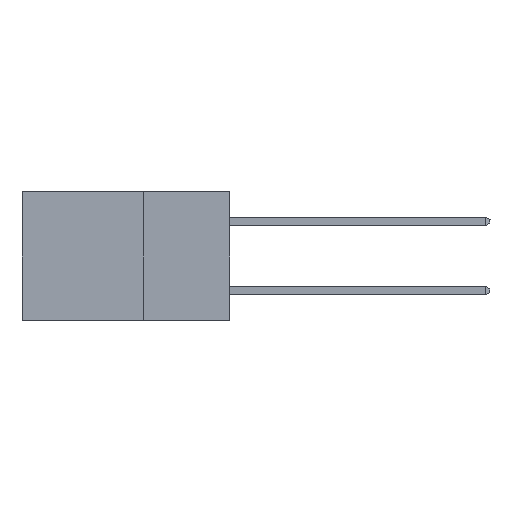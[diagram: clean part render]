
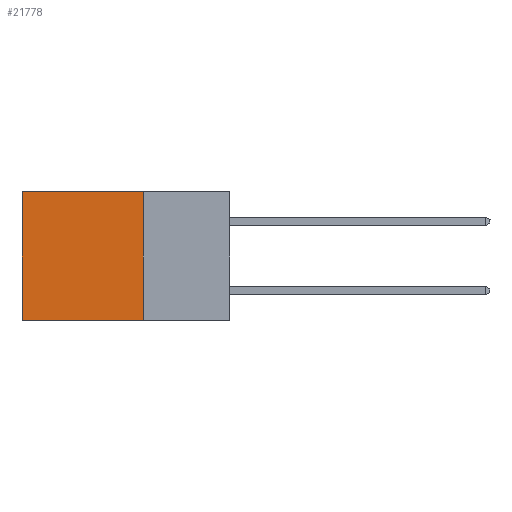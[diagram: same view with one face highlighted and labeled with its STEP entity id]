
A CAD part, left-side view. The second image highlights one B-rep face of the part: STEP entity #21778.
In plain terms, the highlighted planar face has unit normal (-1, 0, 0).
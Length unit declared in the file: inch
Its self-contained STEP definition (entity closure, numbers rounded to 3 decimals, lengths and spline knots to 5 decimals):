
#541 = ORIENTED_EDGE ( 'NONE', *, *, #10721, .F. ) ;
#593 = VERTEX_POINT ( 'NONE', #3258 ) ;
#836 = VECTOR ( 'NONE', #20113, 39.37008 ) ;
#1890 = EDGE_CURVE ( 'NONE', #23855, #11666, #22236, .T. ) ;
#2056 = VECTOR ( 'NONE', #9355, 39.37008 ) ;
#2934 = LINE ( 'NONE', #17889, #4771 ) ;
#3258 = CARTESIAN_POINT ( 'NONE',  ( 0.2615, 0.25, -0.37 ) ) ;
#3886 = CARTESIAN_POINT ( 'NONE',  ( 0.2615, 0.25, 0. ) ) ;
#4771 = VECTOR ( 'NONE', #24038, 39.37008 ) ;
#5005 = PLANE ( 'NONE',  #21907 ) ;
#5134 = LINE ( 'NONE', #14354, #836 ) ;
#5873 = LINE ( 'NONE', #3886, #2056 ) ;
#6566 = CARTESIAN_POINT ( 'NONE',  ( 0.2615, 0.6, -0.37 ) ) ;
#6611 = FACE_OUTER_BOUND ( 'NONE', #23093, .T. ) ;
#7115 = DIRECTION ( 'NONE',  ( 1., 0., 0. ) ) ;
#8564 = ORIENTED_EDGE ( 'NONE', *, *, #1890, .T. ) ;
#9355 = DIRECTION ( 'NONE',  ( 0., 1., 0. ) ) ;
#10398 = ORIENTED_EDGE ( 'NONE', *, *, #10893, .T. ) ;
#10596 = CARTESIAN_POINT ( 'NONE',  ( 0.2615, 0.25, -0.37 ) ) ;
#10721 = EDGE_CURVE ( 'NONE', #11918, #593, #5134, .T. ) ;
#10893 = EDGE_CURVE ( 'NONE', #11918, #23855, #5873, .T. ) ;
#10968 = DIRECTION ( 'NONE',  ( 0., 0., -1. ) ) ;
#11666 = VERTEX_POINT ( 'NONE', #6566 ) ;
#11918 = VERTEX_POINT ( 'NONE', #23057 ) ;
#12061 = CARTESIAN_POINT ( 'NONE',  ( 0.2615, 0.6, 0. ) ) ;
#12595 = DIRECTION ( 'NONE',  ( 0., 0., -1. ) ) ;
#12718 = CARTESIAN_POINT ( 'NONE',  ( 0.2615, 0.6, -0.37 ) ) ;
#14354 = CARTESIAN_POINT ( 'NONE',  ( 0.2615, 0.25, -0.37 ) ) ;
#17889 = CARTESIAN_POINT ( 'NONE',  ( 0.2615, 0.25, -0.37 ) ) ;
#20113 = DIRECTION ( 'NONE',  ( 0., 0., -1. ) ) ;
#20580 = VECTOR ( 'NONE', #10968, 39.37008 ) ;
#21778 = ADVANCED_FACE ( 'NONE', ( #6611 ), #5005, .F. ) ;
#21907 = AXIS2_PLACEMENT_3D ( 'NONE', #10596, #7115, #12595 ) ;
#22236 = LINE ( 'NONE', #12718, #20580 ) ;
#23057 = CARTESIAN_POINT ( 'NONE',  ( 0.2615, 0.25, 0. ) ) ;
#23093 = EDGE_LOOP ( 'NONE', ( #8564, #23282, #541, #10398 ) ) ;
#23282 = ORIENTED_EDGE ( 'NONE', *, *, #24417, .F. ) ;
#23855 = VERTEX_POINT ( 'NONE', #12061 ) ;
#24038 = DIRECTION ( 'NONE',  ( 0., 1., 0. ) ) ;
#24417 = EDGE_CURVE ( 'NONE', #593, #11666, #2934, .T. ) ;
